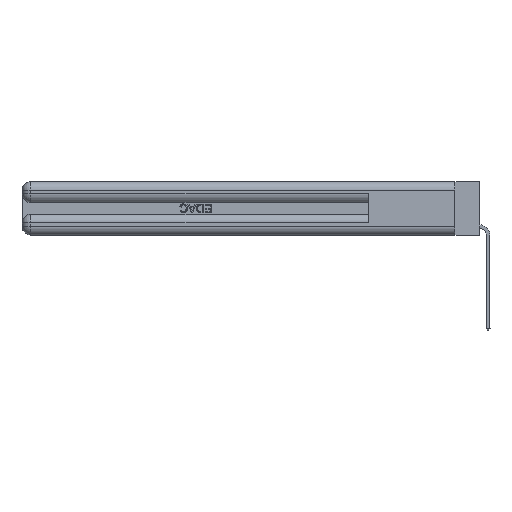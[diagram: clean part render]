
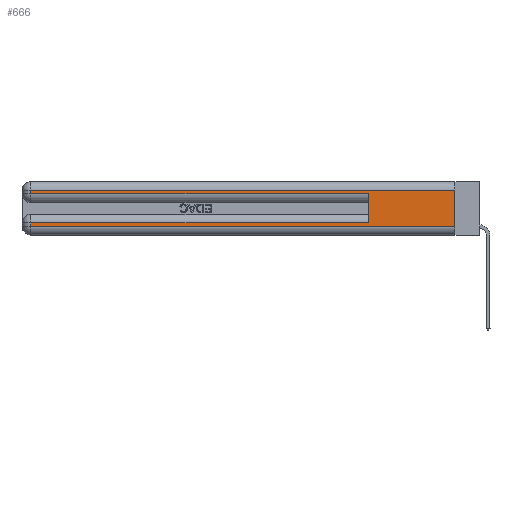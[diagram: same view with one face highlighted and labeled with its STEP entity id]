
A CAD part, left-side view. The second image highlights one B-rep face of the part: STEP entity #666.
In plain terms, the highlighted planar face has unit normal (-1, 0, 0).
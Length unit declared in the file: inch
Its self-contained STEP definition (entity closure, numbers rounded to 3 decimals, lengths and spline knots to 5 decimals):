
#206 = CARTESIAN_POINT ( 'NONE',  ( 0., 2.94, 0.085 ) ) ;
#666 = ADVANCED_FACE ( 'NONE', ( #5799 ), #14156, .F. ) ;
#992 = DIRECTION ( 'NONE',  ( 0., 0., 1. ) ) ;
#1101 = LINE ( 'NONE', #1367, #15472 ) ;
#1219 = EDGE_CURVE ( 'NONE', #1444, #23606, #21451, .T. ) ;
#1367 = CARTESIAN_POINT ( 'NONE',  ( 0., 0., 0.31 ) ) ;
#1437 = DIRECTION ( 'NONE',  ( 0., 0., -1. ) ) ;
#1444 = VERTEX_POINT ( 'NONE', #7345 ) ;
#1599 = ORIENTED_EDGE ( 'NONE', *, *, #12903, .T. ) ;
#1698 = VECTOR ( 'NONE', #18114, 39.37008 ) ;
#3376 = CARTESIAN_POINT ( 'NONE',  ( 0., 0., 0.31 ) ) ;
#3900 = CARTESIAN_POINT ( 'NONE',  ( 0., 0., 0.06 ) ) ;
#4791 = LINE ( 'NONE', #23263, #22770 ) ;
#5068 = DIRECTION ( 'NONE',  ( 0., 1., 0. ) ) ;
#5141 = CARTESIAN_POINT ( 'NONE',  ( 0., 0., 0.285 ) ) ;
#5162 = AXIS2_PLACEMENT_3D ( 'NONE', #24251, #22486, #12236 ) ;
#5799 = FACE_OUTER_BOUND ( 'NONE', #26449, .T. ) ;
#6549 = DIRECTION ( 'NONE',  ( 0., 0., -1. ) ) ;
#7345 = CARTESIAN_POINT ( 'NONE',  ( 0., 2.94, 0.31 ) ) ;
#7862 = CARTESIAN_POINT ( 'NONE',  ( 0., 2.94, 0.285 ) ) ;
#8368 = VERTEX_POINT ( 'NONE', #206 ) ;
#8604 = ORIENTED_EDGE ( 'NONE', *, *, #25197, .T. ) ;
#8898 = DIRECTION ( 'NONE',  ( 0., 0., -1. ) ) ;
#9321 = ORIENTED_EDGE ( 'NONE', *, *, #11554, .F. ) ;
#9377 = DIRECTION ( 'NONE',  ( 0., 1., 0. ) ) ;
#9663 = ORIENTED_EDGE ( 'NONE', *, *, #24222, .T. ) ;
#10119 = VERTEX_POINT ( 'NONE', #17252 ) ;
#10286 = EDGE_CURVE ( 'NONE', #20435, #20718, #24215, .T. ) ;
#11554 = EDGE_CURVE ( 'NONE', #15994, #10119, #4791, .T. ) ;
#12103 = ORIENTED_EDGE ( 'NONE', *, *, #1219, .T. ) ;
#12236 = DIRECTION ( 'NONE',  ( 0., 0., -1. ) ) ;
#12903 = EDGE_CURVE ( 'NONE', #23606, #20718, #23868, .T. ) ;
#13017 = EDGE_CURVE ( 'NONE', #26617, #10119, #18249, .T. ) ;
#13706 = CARTESIAN_POINT ( 'NONE',  ( 0., 0.6, 0.145 ) ) ;
#14156 = PLANE ( 'NONE',  #5162 ) ;
#14826 = VECTOR ( 'NONE', #6549, 39.37008 ) ;
#15163 = CARTESIAN_POINT ( 'NONE',  ( 0., 2.94, 0.37 ) ) ;
#15472 = VECTOR ( 'NONE', #5068, 39.37008 ) ;
#15484 = ORIENTED_EDGE ( 'NONE', *, *, #24190, .T. ) ;
#15937 = CARTESIAN_POINT ( 'NONE',  ( 0., 0., 0.085 ) ) ;
#15994 = VERTEX_POINT ( 'NONE', #3376 ) ;
#16067 = LINE ( 'NONE', #15937, #24596 ) ;
#16287 = CARTESIAN_POINT ( 'NONE',  ( 0., 2.94, 0.06 ) ) ;
#17252 = CARTESIAN_POINT ( 'NONE',  ( 0., 0., 0.06 ) ) ;
#17433 = VECTOR ( 'NONE', #992, 39.37008 ) ;
#17470 = ORIENTED_EDGE ( 'NONE', *, *, #10286, .F. ) ;
#18114 = DIRECTION ( 'NONE',  ( 0., -1., 0. ) ) ;
#18249 = LINE ( 'NONE', #3900, #21475 ) ;
#18935 = VECTOR ( 'NONE', #1437, 39.37008 ) ;
#20176 = CARTESIAN_POINT ( 'NONE',  ( 0., 2.94, 0.37 ) ) ;
#20435 = VERTEX_POINT ( 'NONE', #24994 ) ;
#20718 = VERTEX_POINT ( 'NONE', #25797 ) ;
#21451 = LINE ( 'NONE', #15163, #14826 ) ;
#21475 = VECTOR ( 'NONE', #26597, 39.37008 ) ;
#22486 = DIRECTION ( 'NONE',  ( 1., 0., 0. ) ) ;
#22770 = VECTOR ( 'NONE', #8898, 39.37008 ) ;
#23263 = CARTESIAN_POINT ( 'NONE',  ( 0., 0., 0.37 ) ) ;
#23606 = VERTEX_POINT ( 'NONE', #7862 ) ;
#23868 = LINE ( 'NONE', #5141, #1698 ) ;
#24190 = EDGE_CURVE ( 'NONE', #8368, #26617, #24401, .T. ) ;
#24215 = LINE ( 'NONE', #13706, #17433 ) ;
#24222 = EDGE_CURVE ( 'NONE', #20435, #8368, #16067, .T. ) ;
#24251 = CARTESIAN_POINT ( 'NONE',  ( 0., 0., 0.37 ) ) ;
#24401 = LINE ( 'NONE', #20176, #18935 ) ;
#24596 = VECTOR ( 'NONE', #9377, 39.37008 ) ;
#24994 = CARTESIAN_POINT ( 'NONE',  ( 0., 0.6, 0.085 ) ) ;
#25197 = EDGE_CURVE ( 'NONE', #15994, #1444, #1101, .T. ) ;
#25797 = CARTESIAN_POINT ( 'NONE',  ( 0., 0.6, 0.285 ) ) ;
#26442 = ORIENTED_EDGE ( 'NONE', *, *, #13017, .T. ) ;
#26449 = EDGE_LOOP ( 'NONE', ( #9321, #8604, #12103, #1599, #17470, #9663, #15484, #26442 ) ) ;
#26597 = DIRECTION ( 'NONE',  ( 0., -1., 0. ) ) ;
#26617 = VERTEX_POINT ( 'NONE', #16287 ) ;
